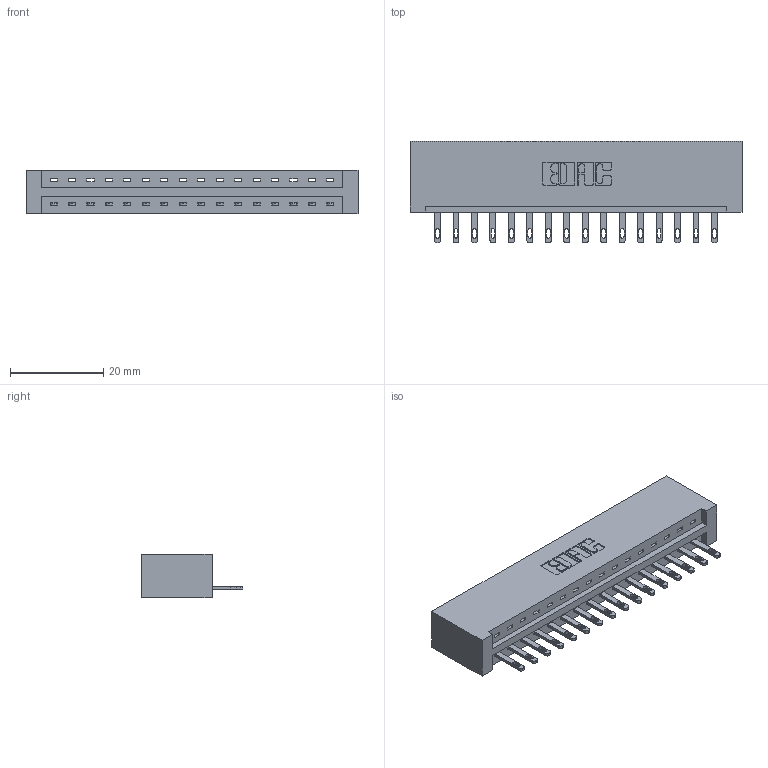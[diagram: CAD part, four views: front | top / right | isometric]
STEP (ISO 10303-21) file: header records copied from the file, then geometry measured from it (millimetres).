
FILE_DESCRIPTION (( 'STEP AP203' ), '1' );
FILE_NAME ('337-016-500-101.STEP', '2019-09-28T17:08:40', ( '' ), ( '' ), 'SwSTEP 2.0', 'SolidWorks 2016', '' );
FILE_SCHEMA (( 'CONFIG_CONTROL_DESIGN' ));
Length unit declared in the file: inch
Products named in the file (3): 337-016-500-101; 345-292-001_345-293-100; 337 Part_No Mounting Lugs
Assembly tree (17 placements, depth 2):
  337-016-500-101
    337 Part_No Mounting Lugs
    345-292-001_345-293-100  x16
Bounding box: 71.27 x 21.85 x 9.4 mm (x, y, z)
Volume: 7830.8 mm3; surface area: 7966.5 mm2
Topology: 17 solids, 17 shells, 1034 faces, 3167 edges, 2110 vertices
Faces by surface type: plane 706, cylinder 328
Entity records: 14909 total; most frequent: CARTESIAN_POINT 2602, ORIENTED_EDGE 2554, DIRECTION 2237, EDGE_CURVE 1277, LINE 1153, VECTOR 1153, VERTEX_POINT 850, AXIS2_PLACEMENT_3D 542
